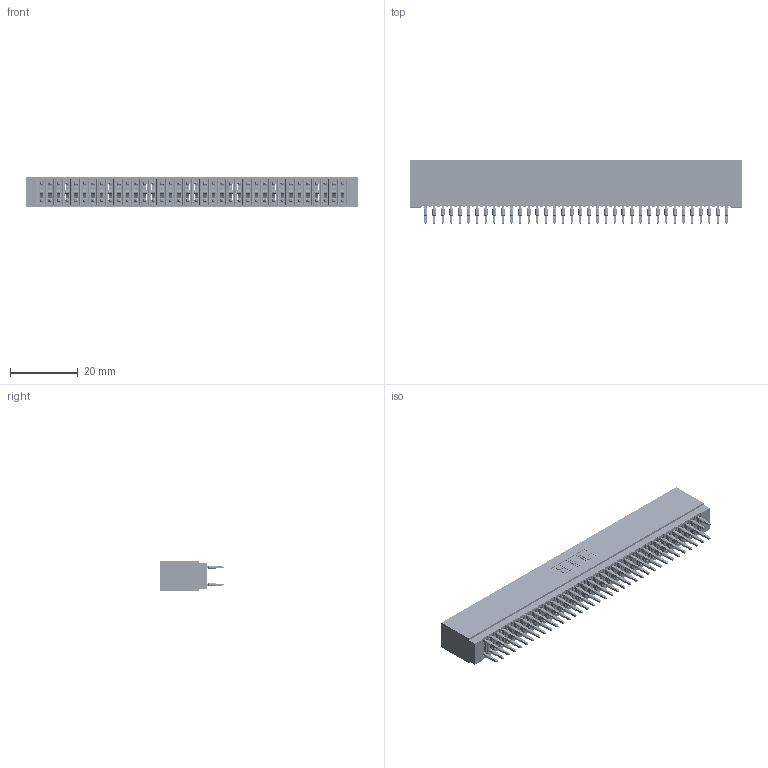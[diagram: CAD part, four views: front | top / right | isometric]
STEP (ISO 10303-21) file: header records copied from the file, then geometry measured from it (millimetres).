
FILE_DESCRIPTION (( 'STEP AP203' ), '1' );
FILE_NAME ('725-072-560-201.STEP', '2026-02-24T18:43:26', ( '' ), ( '' ), 'SwSTEP 2.0', 'SolidWorks 2023', '' );
FILE_SCHEMA (( 'CONFIG_CONTROL_DESIGN' ));
Length unit declared in the file: millimetre
Products named in the file (3): 725 Part_Insulator Option - 01; 745-292-001_560; 725-072-560-201
Assembly tree (73 placements, depth 2):
  725-072-560-201
    725 Part_Insulator Option - 01
    745-292-001_560  x72
Bounding box: 98.04 x 18.8 x 8.89 mm (x, y, z)
Volume: 8071.2 mm3; surface area: 18054.3 mm2
Topology: 73 solids, 73 shells, 7187 faces, 19658 edges, 12480 vertices
Faces by surface type: plane 3727, cylinder 1588, bspline 1440, torus 432
Entity records: 61713 total; most frequent: CARTESIAN_POINT 11209, ORIENTED_EDGE 10632, DIRECTION 9300, EDGE_CURVE 5316, VECTOR 4910, LINE 4910, VERTEX_POINT 3392, AXIS2_PLACEMENT_3D 2195
